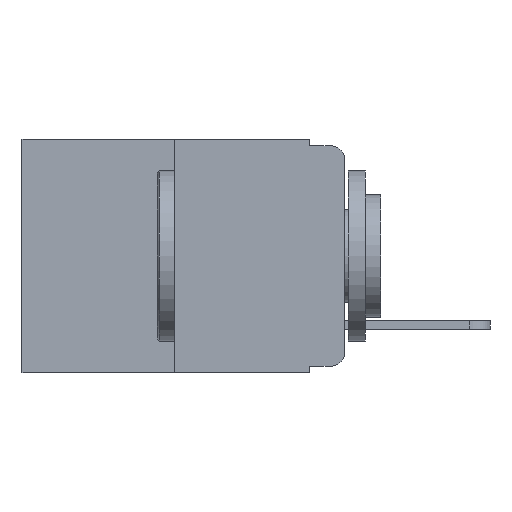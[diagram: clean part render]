
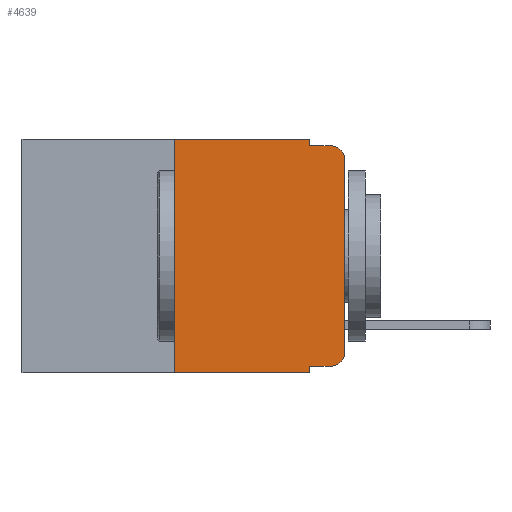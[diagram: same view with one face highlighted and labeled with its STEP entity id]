
A CAD part, left-side view. The second image highlights one B-rep face of the part: STEP entity #4639.
In plain terms, the highlighted planar face has unit normal (-1, 0, 0).
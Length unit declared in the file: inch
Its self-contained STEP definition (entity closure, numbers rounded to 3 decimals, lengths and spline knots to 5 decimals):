
#218 = CARTESIAN_POINT ( 'NONE',  ( 0., 0.25, 0. ) ) ;
#339 = EDGE_CURVE ( 'NONE', #12163, #10177, #14689, .T. ) ;
#430 = LINE ( 'NONE', #15278, #2285 ) ;
#448 = DIRECTION ( 'NONE',  ( 0., -1., 0. ) ) ;
#588 = ORIENTED_EDGE ( 'NONE', *, *, #13132, .T. ) ;
#593 = LINE ( 'NONE', #13330, #7663 ) ;
#610 = AXIS2_PLACEMENT_3D ( 'NONE', #5083, #612, #17338 ) ;
#612 = DIRECTION ( 'NONE',  ( -1., 0., 0. ) ) ;
#778 = AXIS2_PLACEMENT_3D ( 'NONE', #9996, #16286, #2617 ) ;
#808 = ORIENTED_EDGE ( 'NONE', *, *, #10868, .F. ) ;
#1805 = EDGE_CURVE ( 'NONE', #11869, #16861, #10773, .T. ) ;
#1995 = ORIENTED_EDGE ( 'NONE', *, *, #339, .T. ) ;
#2149 = CARTESIAN_POINT ( 'NONE',  ( 0., 0.25, 0. ) ) ;
#2238 = LINE ( 'NONE', #9462, #18548 ) ;
#2285 = VECTOR ( 'NONE', #12308, 39.37008 ) ;
#2305 = ORIENTED_EDGE ( 'NONE', *, *, #12585, .T. ) ;
#2474 = EDGE_CURVE ( 'NONE', #10177, #10854, #3658, .T. ) ;
#2616 = DIRECTION ( 'NONE',  ( 0., 0., -1. ) ) ;
#2617 = DIRECTION ( 'NONE',  ( 0., 0., -1. ) ) ;
#3658 = LINE ( 'NONE', #12955, #17133 ) ;
#3660 = VERTEX_POINT ( 'NONE', #5686 ) ;
#3848 = ORIENTED_EDGE ( 'NONE', *, *, #16842, .T. ) ;
#4151 = CARTESIAN_POINT ( 'NONE',  ( 0., 0., -0.313 ) ) ;
#4574 = DIRECTION ( 'NONE',  ( 0., -1., 0. ) ) ;
#4639 = ADVANCED_FACE ( 'NONE', ( #6930 ), #11653, .F. ) ;
#5083 = CARTESIAN_POINT ( 'NONE',  ( 0., 0.02, -0.313 ) ) ;
#5577 = DIRECTION ( 'NONE',  ( 0., 0., -1. ) ) ;
#5686 = CARTESIAN_POINT ( 'NONE',  ( 0., 0.02, -0.01 ) ) ;
#6043 = CARTESIAN_POINT ( 'NONE',  ( 0., 0.473, -0.343 ) ) ;
#6327 = ORIENTED_EDGE ( 'NONE', *, *, #19234, .F. ) ;
#6900 = CARTESIAN_POINT ( 'NONE',  ( 0., 0.25, -0.343 ) ) ;
#6930 = FACE_OUTER_BOUND ( 'NONE', #16588, .T. ) ;
#7197 = CARTESIAN_POINT ( 'NONE',  ( 0., 0.473, 0. ) ) ;
#7253 = CARTESIAN_POINT ( 'NONE',  ( 0., 0., -0.03 ) ) ;
#7314 = CARTESIAN_POINT ( 'NONE',  ( 0., 0.051, 0. ) ) ;
#7663 = VECTOR ( 'NONE', #13397, 39.37008 ) ;
#8362 = ORIENTED_EDGE ( 'NONE', *, *, #1805, .F. ) ;
#8522 = CIRCLE ( 'NONE', #778, 0.02 ) ;
#9349 = CARTESIAN_POINT ( 'NONE',  ( 0., 0.051, -0.343 ) ) ;
#9367 = EDGE_CURVE ( 'NONE', #12432, #3660, #2238, .T. ) ;
#9462 = CARTESIAN_POINT ( 'NONE',  ( 0., 0.051, -0.01 ) ) ;
#9542 = ORIENTED_EDGE ( 'NONE', *, *, #18709, .F. ) ;
#9550 = VECTOR ( 'NONE', #15486, 39.37008 ) ;
#9870 = AXIS2_PLACEMENT_3D ( 'NONE', #7197, #13251, #2616 ) ;
#9996 = CARTESIAN_POINT ( 'NONE',  ( 0., 0.02, -0.03 ) ) ;
#10177 = VERTEX_POINT ( 'NONE', #4151 ) ;
#10773 = LINE ( 'NONE', #7314, #12903 ) ;
#10854 = VERTEX_POINT ( 'NONE', #7253 ) ;
#10868 = EDGE_CURVE ( 'NONE', #14606, #12432, #19395, .T. ) ;
#11451 = DIRECTION ( 'NONE',  ( 0., 0., 1. ) ) ;
#11653 = PLANE ( 'NONE',  #9870 ) ;
#11851 = VERTEX_POINT ( 'NONE', #6900 ) ;
#11869 = VERTEX_POINT ( 'NONE', #16055 ) ;
#12163 = VERTEX_POINT ( 'NONE', #16784 ) ;
#12308 = DIRECTION ( 'NONE',  ( 0., -1., 0. ) ) ;
#12432 = VERTEX_POINT ( 'NONE', #12929 ) ;
#12585 = EDGE_CURVE ( 'NONE', #10854, #3660, #8522, .T. ) ;
#12815 = VERTEX_POINT ( 'NONE', #218 ) ;
#12903 = VECTOR ( 'NONE', #14827, 39.37008 ) ;
#12929 = CARTESIAN_POINT ( 'NONE',  ( 0., 0.051, -0.01 ) ) ;
#12955 = CARTESIAN_POINT ( 'NONE',  ( 0., 0., 0. ) ) ;
#13132 = EDGE_CURVE ( 'NONE', #11851, #16861, #16021, .T. ) ;
#13251 = DIRECTION ( 'NONE',  ( 1., 0., 0. ) ) ;
#13330 = CARTESIAN_POINT ( 'NONE',  ( 0., 0.473, 0. ) ) ;
#13397 = DIRECTION ( 'NONE',  ( 0., -1., 0. ) ) ;
#14606 = VERTEX_POINT ( 'NONE', #17447 ) ;
#14689 = CIRCLE ( 'NONE', #610, 0.02 ) ;
#14827 = DIRECTION ( 'NONE',  ( 0., 0., -1. ) ) ;
#15278 = CARTESIAN_POINT ( 'NONE',  ( 0., 0.051, -0.333 ) ) ;
#15434 = VECTOR ( 'NONE', #5577, 39.37008 ) ;
#15486 = DIRECTION ( 'NONE',  ( 0., 0., 1. ) ) ;
#16021 = LINE ( 'NONE', #6043, #17219 ) ;
#16055 = CARTESIAN_POINT ( 'NONE',  ( 0., 0.051, -0.333 ) ) ;
#16286 = DIRECTION ( 'NONE',  ( -1., 0., 0. ) ) ;
#16588 = EDGE_LOOP ( 'NONE', ( #17207, #2305, #16644, #808, #6327, #9542, #588, #8362, #3848, #1995 ) ) ;
#16644 = ORIENTED_EDGE ( 'NONE', *, *, #9367, .F. ) ;
#16784 = CARTESIAN_POINT ( 'NONE',  ( 0., 0.02, -0.333 ) ) ;
#16842 = EDGE_CURVE ( 'NONE', #11869, #12163, #430, .T. ) ;
#16861 = VERTEX_POINT ( 'NONE', #9349 ) ;
#17133 = VECTOR ( 'NONE', #11451, 39.37008 ) ;
#17207 = ORIENTED_EDGE ( 'NONE', *, *, #2474, .T. ) ;
#17219 = VECTOR ( 'NONE', #4574, 39.37008 ) ;
#17338 = DIRECTION ( 'NONE',  ( 0., 0., -1. ) ) ;
#17447 = CARTESIAN_POINT ( 'NONE',  ( 0., 0.051, 0. ) ) ;
#17552 = LINE ( 'NONE', #2149, #9550 ) ;
#17861 = CARTESIAN_POINT ( 'NONE',  ( 0., 0.051, 0. ) ) ;
#18548 = VECTOR ( 'NONE', #448, 39.37008 ) ;
#18709 = EDGE_CURVE ( 'NONE', #11851, #12815, #17552, .T. ) ;
#19234 = EDGE_CURVE ( 'NONE', #12815, #14606, #593, .T. ) ;
#19395 = LINE ( 'NONE', #17861, #15434 ) ;
